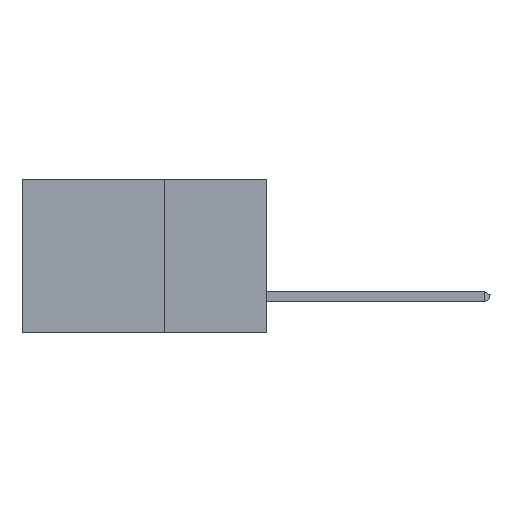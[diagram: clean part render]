
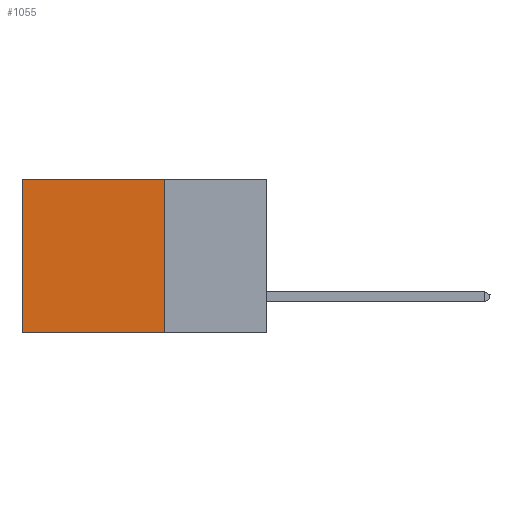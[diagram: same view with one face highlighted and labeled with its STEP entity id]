
A CAD part, left-side view. The second image highlights one B-rep face of the part: STEP entity #1055.
In plain terms, the highlighted planar face has unit normal (-1, 0, 0).
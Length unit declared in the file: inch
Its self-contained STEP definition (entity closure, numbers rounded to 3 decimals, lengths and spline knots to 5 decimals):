
#941 = VERTEX_POINT ( 'NONE', #14652 ) ;
#973 = PLANE ( 'NONE',  #6858 ) ;
#1055 = ADVANCED_FACE ( 'NONE', ( #17140 ), #973, .F. ) ;
#1073 = CARTESIAN_POINT ( 'NONE',  ( 0.2875, 0.25, -0.375 ) ) ;
#2525 = DIRECTION ( 'NONE',  ( 1., 0., 0. ) ) ;
#2545 = VECTOR ( 'NONE', #11968, 39.37008 ) ;
#3668 = DIRECTION ( 'NONE',  ( 0., 0., -1. ) ) ;
#4562 = CARTESIAN_POINT ( 'NONE',  ( 0.2875, 0.6, -0.375 ) ) ;
#5272 = CARTESIAN_POINT ( 'NONE',  ( 0.2875, 0.25, -0.375 ) ) ;
#6180 = VECTOR ( 'NONE', #3668, 39.37008 ) ;
#6460 = CARTESIAN_POINT ( 'NONE',  ( 0.2875, 0.25, 0. ) ) ;
#6499 = EDGE_CURVE ( 'NONE', #13064, #6577, #16464, .T. ) ;
#6577 = VERTEX_POINT ( 'NONE', #17559 ) ;
#6814 = ORIENTED_EDGE ( 'NONE', *, *, #6499, .T. ) ;
#6858 = AXIS2_PLACEMENT_3D ( 'NONE', #5272, #2525, #12256 ) ;
#7751 = DIRECTION ( 'NONE',  ( 0., 0., -1. ) ) ;
#8957 = DIRECTION ( 'NONE',  ( 0., 1., 0. ) ) ;
#9060 = ORIENTED_EDGE ( 'NONE', *, *, #11783, .F. ) ;
#9185 = VECTOR ( 'NONE', #8957, 39.37008 ) ;
#10628 = VECTOR ( 'NONE', #7751, 39.37008 ) ;
#10859 = LINE ( 'NONE', #11761, #10628 ) ;
#10980 = EDGE_LOOP ( 'NONE', ( #12525, #9060, #15293, #6814 ) ) ;
#11360 = EDGE_CURVE ( 'NONE', #13064, #941, #11802, .T. ) ;
#11761 = CARTESIAN_POINT ( 'NONE',  ( 0.2875, 0.6, -0.375 ) ) ;
#11783 = EDGE_CURVE ( 'NONE', #941, #14463, #14209, .T. ) ;
#11802 = LINE ( 'NONE', #1073, #6180 ) ;
#11968 = DIRECTION ( 'NONE',  ( 0., 1., 0. ) ) ;
#12256 = DIRECTION ( 'NONE',  ( 0., 0., -1. ) ) ;
#12525 = ORIENTED_EDGE ( 'NONE', *, *, #17326, .T. ) ;
#12975 = CARTESIAN_POINT ( 'NONE',  ( 0.2875, 0.25, 0. ) ) ;
#13064 = VERTEX_POINT ( 'NONE', #12975 ) ;
#14209 = LINE ( 'NONE', #17098, #9185 ) ;
#14463 = VERTEX_POINT ( 'NONE', #4562 ) ;
#14652 = CARTESIAN_POINT ( 'NONE',  ( 0.2875, 0.25, -0.375 ) ) ;
#15293 = ORIENTED_EDGE ( 'NONE', *, *, #11360, .F. ) ;
#16464 = LINE ( 'NONE', #6460, #2545 ) ;
#17098 = CARTESIAN_POINT ( 'NONE',  ( 0.2875, 0.25, -0.375 ) ) ;
#17140 = FACE_OUTER_BOUND ( 'NONE', #10980, .T. ) ;
#17326 = EDGE_CURVE ( 'NONE', #6577, #14463, #10859, .T. ) ;
#17559 = CARTESIAN_POINT ( 'NONE',  ( 0.2875, 0.6, 0. ) ) ;
